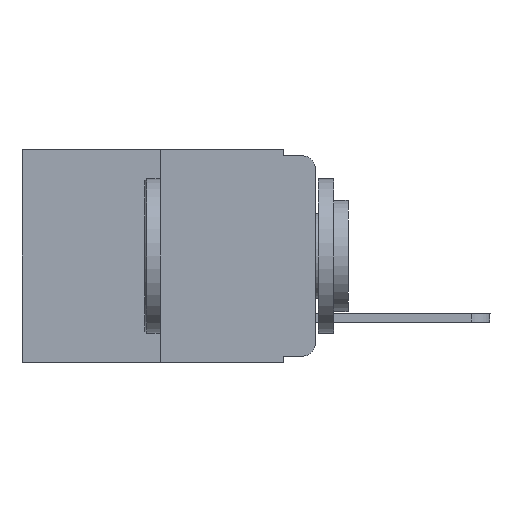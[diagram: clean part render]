
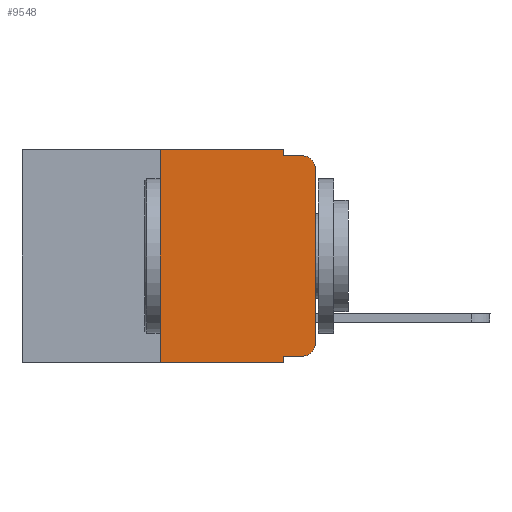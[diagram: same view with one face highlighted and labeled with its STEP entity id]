
A CAD part, left-side view. The second image highlights one B-rep face of the part: STEP entity #9548.
In plain terms, the highlighted planar face has unit normal (-1, 0, 0).
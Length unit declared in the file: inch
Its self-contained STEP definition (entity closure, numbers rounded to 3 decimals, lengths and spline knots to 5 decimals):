
#303 = DIRECTION ( 'NONE',  ( 0., -1., 0. ) ) ;
#373 = VECTOR ( 'NONE', #5726, 39.37008 ) ;
#411 = CARTESIAN_POINT ( 'NONE',  ( 0., 0.473, 0. ) ) ;
#519 = VERTEX_POINT ( 'NONE', #12034 ) ;
#938 = DIRECTION ( 'NONE',  ( 0., 0., -1. ) ) ;
#1455 = VECTOR ( 'NONE', #9787, 39.37008 ) ;
#1467 = CARTESIAN_POINT ( 'NONE',  ( 0., 0.02, -0.01 ) ) ;
#1487 = CARTESIAN_POINT ( 'NONE',  ( 0., 0.051, -0.333 ) ) ;
#1564 = CARTESIAN_POINT ( 'NONE',  ( 0., 0., -0.313 ) ) ;
#1621 = ORIENTED_EDGE ( 'NONE', *, *, #17778, .T. ) ;
#1732 = EDGE_CURVE ( 'NONE', #13509, #4834, #14219, .T. ) ;
#2458 = CARTESIAN_POINT ( 'NONE',  ( 0., 0.02, -0.333 ) ) ;
#2585 = EDGE_CURVE ( 'NONE', #6724, #4950, #12895, .T. ) ;
#2682 = CARTESIAN_POINT ( 'NONE',  ( 0., 0., 0. ) ) ;
#2780 = ORIENTED_EDGE ( 'NONE', *, *, #2585, .F. ) ;
#2856 = CIRCLE ( 'NONE', #13042, 0.02 ) ;
#2899 = VECTOR ( 'NONE', #303, 39.37008 ) ;
#3479 = CIRCLE ( 'NONE', #4050, 0.02 ) ;
#4050 = AXIS2_PLACEMENT_3D ( 'NONE', #13651, #12133, #9491 ) ;
#4130 = ORIENTED_EDGE ( 'NONE', *, *, #15571, .F. ) ;
#4393 = EDGE_CURVE ( 'NONE', #519, #9672, #2856, .T. ) ;
#4419 = LINE ( 'NONE', #1487, #2899 ) ;
#4513 = VERTEX_POINT ( 'NONE', #1564 ) ;
#4834 = VERTEX_POINT ( 'NONE', #16202 ) ;
#4888 = DIRECTION ( 'NONE',  ( 0., 0., -1. ) ) ;
#4950 = VERTEX_POINT ( 'NONE', #17823 ) ;
#5141 = AXIS2_PLACEMENT_3D ( 'NONE', #9164, #6439, #4888 ) ;
#5541 = DIRECTION ( 'NONE',  ( 0., -1., 0. ) ) ;
#5575 = LINE ( 'NONE', #12488, #13392 ) ;
#5726 = DIRECTION ( 'NONE',  ( 0., 0., 1. ) ) ;
#6013 = ORIENTED_EDGE ( 'NONE', *, *, #11449, .F. ) ;
#6299 = EDGE_CURVE ( 'NONE', #6795, #9672, #9543, .T. ) ;
#6439 = DIRECTION ( 'NONE',  ( 1., 0., 0. ) ) ;
#6568 = LINE ( 'NONE', #13636, #7809 ) ;
#6724 = VERTEX_POINT ( 'NONE', #11989 ) ;
#6795 = VERTEX_POINT ( 'NONE', #13768 ) ;
#6814 = LINE ( 'NONE', #2682, #373 ) ;
#7031 = CARTESIAN_POINT ( 'NONE',  ( 0., 0.051, -0.333 ) ) ;
#7581 = VECTOR ( 'NONE', #5541, 39.37008 ) ;
#7662 = ORIENTED_EDGE ( 'NONE', *, *, #6299, .F. ) ;
#7809 = VECTOR ( 'NONE', #16528, 39.37008 ) ;
#8264 = CARTESIAN_POINT ( 'NONE',  ( 0., 0.051, -0.01 ) ) ;
#8296 = DIRECTION ( 'NONE',  ( 0., 0., 1. ) ) ;
#8412 = CARTESIAN_POINT ( 'NONE',  ( 0., 0.051, 0. ) ) ;
#8808 = DIRECTION ( 'NONE',  ( 0., -1., 0. ) ) ;
#9082 = ORIENTED_EDGE ( 'NONE', *, *, #4393, .T. ) ;
#9164 = CARTESIAN_POINT ( 'NONE',  ( 0., 0.473, 0. ) ) ;
#9491 = DIRECTION ( 'NONE',  ( 0., 0., -1. ) ) ;
#9543 = LINE ( 'NONE', #8264, #7581 ) ;
#9548 = ADVANCED_FACE ( 'NONE', ( #10555 ), #17237, .F. ) ;
#9672 = VERTEX_POINT ( 'NONE', #1467 ) ;
#9787 = DIRECTION ( 'NONE',  ( 0., 0., -1. ) ) ;
#10168 = CARTESIAN_POINT ( 'NONE',  ( 0., 0.473, -0.343 ) ) ;
#10555 = FACE_OUTER_BOUND ( 'NONE', #16051, .T. ) ;
#10865 = ORIENTED_EDGE ( 'NONE', *, *, #1732, .T. ) ;
#11449 = EDGE_CURVE ( 'NONE', #15562, #4834, #6568, .T. ) ;
#11954 = VECTOR ( 'NONE', #8808, 39.37008 ) ;
#11989 = CARTESIAN_POINT ( 'NONE',  ( 0., 0.25, 0. ) ) ;
#12034 = CARTESIAN_POINT ( 'NONE',  ( 0., 0., -0.03 ) ) ;
#12133 = DIRECTION ( 'NONE',  ( -1., 0., 0. ) ) ;
#12488 = CARTESIAN_POINT ( 'NONE',  ( 0., 0.25, 0. ) ) ;
#12895 = LINE ( 'NONE', #411, #11954 ) ;
#12966 = DIRECTION ( 'NONE',  ( 0., -1., 0. ) ) ;
#13042 = AXIS2_PLACEMENT_3D ( 'NONE', #16222, #17749, #938 ) ;
#13392 = VECTOR ( 'NONE', #8296, 39.37008 ) ;
#13509 = VERTEX_POINT ( 'NONE', #17054 ) ;
#13636 = CARTESIAN_POINT ( 'NONE',  ( 0., 0.051, 0. ) ) ;
#13651 = CARTESIAN_POINT ( 'NONE',  ( 0., 0.02, -0.313 ) ) ;
#13768 = CARTESIAN_POINT ( 'NONE',  ( 0., 0.051, -0.01 ) ) ;
#13887 = EDGE_CURVE ( 'NONE', #15406, #4513, #3479, .T. ) ;
#13922 = ORIENTED_EDGE ( 'NONE', *, *, #14606, .T. ) ;
#14203 = LINE ( 'NONE', #8412, #1455 ) ;
#14219 = LINE ( 'NONE', #10168, #16910 ) ;
#14606 = EDGE_CURVE ( 'NONE', #15562, #15406, #4419, .T. ) ;
#15115 = EDGE_CURVE ( 'NONE', #4950, #6795, #14203, .T. ) ;
#15406 = VERTEX_POINT ( 'NONE', #2458 ) ;
#15562 = VERTEX_POINT ( 'NONE', #7031 ) ;
#15571 = EDGE_CURVE ( 'NONE', #13509, #6724, #5575, .T. ) ;
#15976 = ORIENTED_EDGE ( 'NONE', *, *, #13887, .T. ) ;
#16051 = EDGE_LOOP ( 'NONE', ( #1621, #9082, #7662, #17610, #2780, #4130, #10865, #6013, #13922, #15976 ) ) ;
#16202 = CARTESIAN_POINT ( 'NONE',  ( 0., 0.051, -0.343 ) ) ;
#16222 = CARTESIAN_POINT ( 'NONE',  ( 0., 0.02, -0.03 ) ) ;
#16528 = DIRECTION ( 'NONE',  ( 0., 0., -1. ) ) ;
#16910 = VECTOR ( 'NONE', #12966, 39.37008 ) ;
#17054 = CARTESIAN_POINT ( 'NONE',  ( 0., 0.25, -0.343 ) ) ;
#17237 = PLANE ( 'NONE',  #5141 ) ;
#17610 = ORIENTED_EDGE ( 'NONE', *, *, #15115, .F. ) ;
#17749 = DIRECTION ( 'NONE',  ( -1., 0., 0. ) ) ;
#17778 = EDGE_CURVE ( 'NONE', #4513, #519, #6814, .T. ) ;
#17823 = CARTESIAN_POINT ( 'NONE',  ( 0., 0.051, 0. ) ) ;
